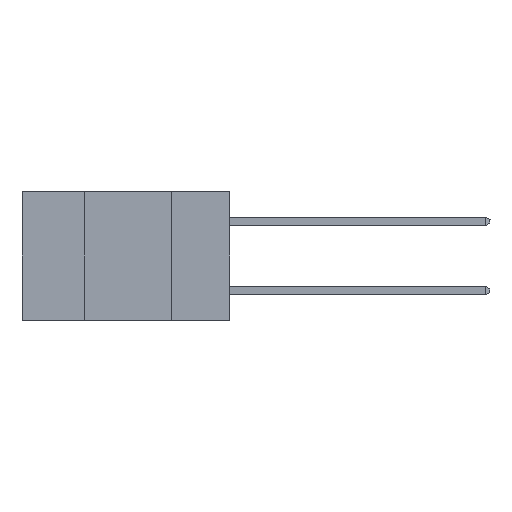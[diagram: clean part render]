
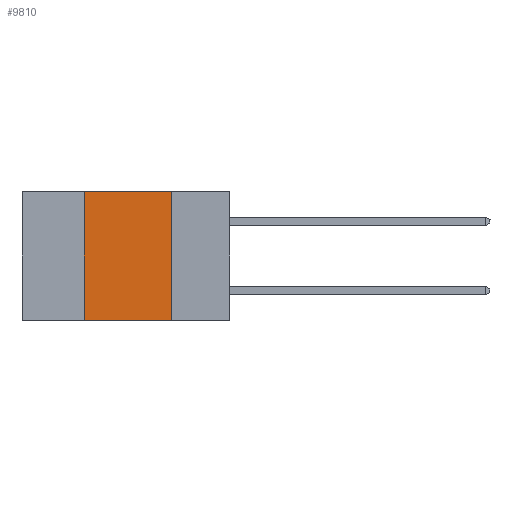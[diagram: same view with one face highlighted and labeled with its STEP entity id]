
A CAD part, left-side view. The second image highlights one B-rep face of the part: STEP entity #9810.
In plain terms, the highlighted planar face has unit normal (-1, 0, 0).
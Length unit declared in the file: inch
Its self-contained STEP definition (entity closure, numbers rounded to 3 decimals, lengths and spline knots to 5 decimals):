
#969 = LINE ( 'NONE', #5312, #1012 ) ;
#1012 = VECTOR ( 'NONE', #1057, 39.37008 ) ;
#1057 = DIRECTION ( 'NONE',  ( 0., -1., 0. ) ) ;
#1373 = CARTESIAN_POINT ( 'NONE',  ( 0., 0.42, -0.37 ) ) ;
#2424 = CARTESIAN_POINT ( 'NONE',  ( 0., 0.42, -0.37 ) ) ;
#2442 = DIRECTION ( 'NONE',  ( 1., 0., 0. ) ) ;
#2781 = ORIENTED_EDGE ( 'NONE', *, *, #3386, .F. ) ;
#2797 = ORIENTED_EDGE ( 'NONE', *, *, #15943, .T. ) ;
#3386 = EDGE_CURVE ( 'NONE', #4236, #9588, #5845, .T. ) ;
#3701 = EDGE_LOOP ( 'NONE', ( #2781, #7097, #10263, #2797 ) ) ;
#4236 = VERTEX_POINT ( 'NONE', #9555 ) ;
#4966 = LINE ( 'NONE', #1373, #12611 ) ;
#5037 = PLANE ( 'NONE',  #11430 ) ;
#5120 = CARTESIAN_POINT ( 'NONE',  ( 0., 0.6, 0. ) ) ;
#5312 = CARTESIAN_POINT ( 'NONE',  ( 0., 0.6, -0.37 ) ) ;
#5673 = VECTOR ( 'NONE', #7185, 39.37008 ) ;
#5845 = LINE ( 'NONE', #16985, #5673 ) ;
#6227 = DIRECTION ( 'NONE',  ( 0., -1., 0. ) ) ;
#6340 = VECTOR ( 'NONE', #6227, 39.37008 ) ;
#6575 = LINE ( 'NONE', #14515, #6340 ) ;
#7097 = ORIENTED_EDGE ( 'NONE', *, *, #12917, .F. ) ;
#7185 = DIRECTION ( 'NONE',  ( 0., 0., -1. ) ) ;
#9555 = CARTESIAN_POINT ( 'NONE',  ( 0., 0.17, 0. ) ) ;
#9588 = VERTEX_POINT ( 'NONE', #12533 ) ;
#9810 = ADVANCED_FACE ( 'NONE', ( #13153 ), #5037, .F. ) ;
#10263 = ORIENTED_EDGE ( 'NONE', *, *, #13313, .F. ) ;
#10903 = DIRECTION ( 'NONE',  ( 0., 0., 1. ) ) ;
#11430 = AXIS2_PLACEMENT_3D ( 'NONE', #5120, #2442, #16087 ) ;
#11599 = VERTEX_POINT ( 'NONE', #2424 ) ;
#12533 = CARTESIAN_POINT ( 'NONE',  ( 0., 0.17, -0.37 ) ) ;
#12611 = VECTOR ( 'NONE', #10903, 39.37008 ) ;
#12911 = VERTEX_POINT ( 'NONE', #15858 ) ;
#12917 = EDGE_CURVE ( 'NONE', #12911, #4236, #6575, .T. ) ;
#13153 = FACE_OUTER_BOUND ( 'NONE', #3701, .T. ) ;
#13313 = EDGE_CURVE ( 'NONE', #11599, #12911, #4966, .T. ) ;
#14515 = CARTESIAN_POINT ( 'NONE',  ( 0., 0.6, 0. ) ) ;
#15858 = CARTESIAN_POINT ( 'NONE',  ( 0., 0.42, 0. ) ) ;
#15943 = EDGE_CURVE ( 'NONE', #11599, #9588, #969, .T. ) ;
#16087 = DIRECTION ( 'NONE',  ( 0., 0., -1. ) ) ;
#16985 = CARTESIAN_POINT ( 'NONE',  ( 0., 0.17, -0.37 ) ) ;
